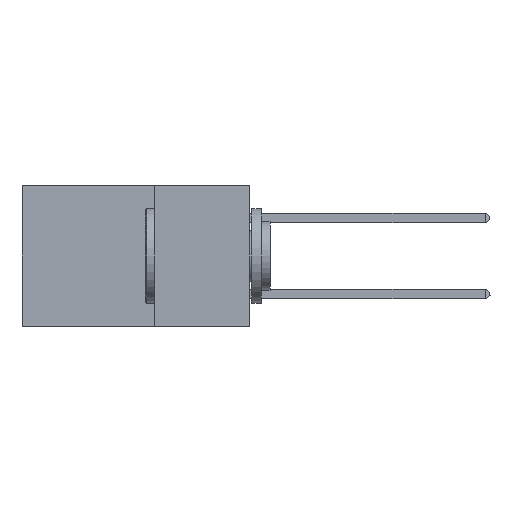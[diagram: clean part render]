
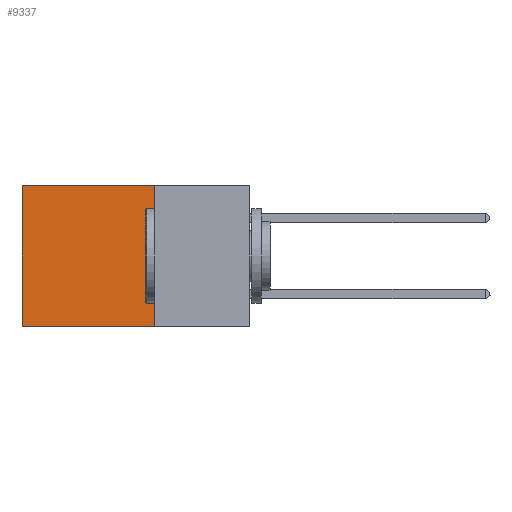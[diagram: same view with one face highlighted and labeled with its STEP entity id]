
A CAD part, left-side view. The second image highlights one B-rep face of the part: STEP entity #9337.
In plain terms, the highlighted planar face has unit normal (-1, 0, 0).
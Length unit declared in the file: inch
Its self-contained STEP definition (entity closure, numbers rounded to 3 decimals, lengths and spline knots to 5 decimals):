
#804 = VERTEX_POINT ( 'NONE', #7977 ) ;
#1075 = EDGE_LOOP ( 'NONE', ( #1760, #10832, #6073, #1822 ) ) ;
#1159 = LINE ( 'NONE', #1465, #4786 ) ;
#1185 = EDGE_CURVE ( 'NONE', #2946, #9526, #16320, .T. ) ;
#1465 = CARTESIAN_POINT ( 'NONE',  ( 0.2875, 0.25, 0. ) ) ;
#1760 = ORIENTED_EDGE ( 'NONE', *, *, #8001, .T. ) ;
#1822 = ORIENTED_EDGE ( 'NONE', *, *, #5092, .T. ) ;
#2703 = CARTESIAN_POINT ( 'NONE',  ( 0.2875, 0.25, 0. ) ) ;
#2946 = VERTEX_POINT ( 'NONE', #13720 ) ;
#4122 = CARTESIAN_POINT ( 'NONE',  ( 0.2875, 0.6, 0. ) ) ;
#4138 = PLANE ( 'NONE',  #4956 ) ;
#4406 = VECTOR ( 'NONE', #7116, 39.37008 ) ;
#4493 = DIRECTION ( 'NONE',  ( 0., 1., 0. ) ) ;
#4494 = VECTOR ( 'NONE', #11158, 39.37008 ) ;
#4543 = VERTEX_POINT ( 'NONE', #10803 ) ;
#4786 = VECTOR ( 'NONE', #4493, 39.37008 ) ;
#4956 = AXIS2_PLACEMENT_3D ( 'NONE', #2703, #14617, #5722 ) ;
#5092 = EDGE_CURVE ( 'NONE', #4543, #804, #1159, .T. ) ;
#5722 = DIRECTION ( 'NONE',  ( 0., 0., -1. ) ) ;
#6073 = ORIENTED_EDGE ( 'NONE', *, *, #11202, .F. ) ;
#7116 = DIRECTION ( 'NONE',  ( 0., 0., -1. ) ) ;
#7977 = CARTESIAN_POINT ( 'NONE',  ( 0.2875, 0.6, 0. ) ) ;
#8001 = EDGE_CURVE ( 'NONE', #804, #9526, #9285, .T. ) ;
#9285 = LINE ( 'NONE', #4122, #4406 ) ;
#9337 = ADVANCED_FACE ( 'NONE', ( #18231 ), #4138, .F. ) ;
#9526 = VERTEX_POINT ( 'NONE', #13562 ) ;
#9608 = LINE ( 'NONE', #15511, #17003 ) ;
#10803 = CARTESIAN_POINT ( 'NONE',  ( 0.2875, 0.25, 0. ) ) ;
#10832 = ORIENTED_EDGE ( 'NONE', *, *, #1185, .F. ) ;
#11121 = CARTESIAN_POINT ( 'NONE',  ( 0.2875, 0.25, -0.37 ) ) ;
#11158 = DIRECTION ( 'NONE',  ( 0., 1., 0. ) ) ;
#11202 = EDGE_CURVE ( 'NONE', #4543, #2946, #9608, .T. ) ;
#13562 = CARTESIAN_POINT ( 'NONE',  ( 0.2875, 0.6, -0.37 ) ) ;
#13720 = CARTESIAN_POINT ( 'NONE',  ( 0.2875, 0.25, -0.37 ) ) ;
#14617 = DIRECTION ( 'NONE',  ( 1., 0., 0. ) ) ;
#15511 = CARTESIAN_POINT ( 'NONE',  ( 0.2875, 0.25, 0. ) ) ;
#16320 = LINE ( 'NONE', #11121, #4494 ) ;
#16957 = DIRECTION ( 'NONE',  ( 0., 0., -1. ) ) ;
#17003 = VECTOR ( 'NONE', #16957, 39.37008 ) ;
#18231 = FACE_OUTER_BOUND ( 'NONE', #1075, .T. ) ;
